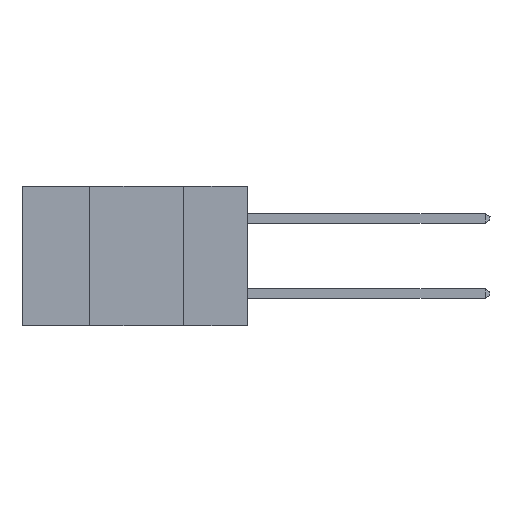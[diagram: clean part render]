
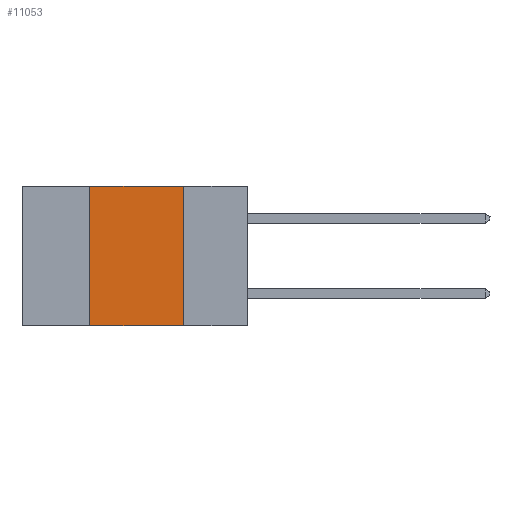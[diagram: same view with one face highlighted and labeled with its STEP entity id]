
A CAD part, left-side view. The second image highlights one B-rep face of the part: STEP entity #11053.
In plain terms, the highlighted planar face has unit normal (-1, 0, 0).
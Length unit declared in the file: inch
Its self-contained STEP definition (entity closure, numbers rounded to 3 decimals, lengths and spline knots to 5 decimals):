
#261 = DIRECTION ( 'NONE',  ( 0., -1., 0. ) ) ;
#822 = CARTESIAN_POINT ( 'NONE',  ( 0., 0.42, 0. ) ) ;
#1198 = VECTOR ( 'NONE', #261, 39.37008 ) ;
#1407 = DIRECTION ( 'NONE',  ( 0., 0., -1. ) ) ;
#1508 = EDGE_CURVE ( 'NONE', #2218, #7993, #6238, .T. ) ;
#2218 = VERTEX_POINT ( 'NONE', #10635 ) ;
#2690 = VECTOR ( 'NONE', #10118, 39.37008 ) ;
#2899 = LINE ( 'NONE', #6430, #2690 ) ;
#2965 = ORIENTED_EDGE ( 'NONE', *, *, #9736, .F. ) ;
#3359 = DIRECTION ( 'NONE',  ( 0., 0., 1. ) ) ;
#4343 = AXIS2_PLACEMENT_3D ( 'NONE', #10699, #7095, #15680 ) ;
#4502 = VERTEX_POINT ( 'NONE', #822 ) ;
#4747 = EDGE_CURVE ( 'NONE', #8510, #7993, #2899, .T. ) ;
#5065 = EDGE_CURVE ( 'NONE', #4502, #2218, #14714, .T. ) ;
#6238 = LINE ( 'NONE', #11136, #9952 ) ;
#6390 = ORIENTED_EDGE ( 'NONE', *, *, #1508, .F. ) ;
#6430 = CARTESIAN_POINT ( 'NONE',  ( 0., 0.6, -0.37 ) ) ;
#6575 = VECTOR ( 'NONE', #3359, 39.37008 ) ;
#6958 = LINE ( 'NONE', #9565, #6575 ) ;
#7030 = ORIENTED_EDGE ( 'NONE', *, *, #4747, .T. ) ;
#7095 = DIRECTION ( 'NONE',  ( 1., 0., 0. ) ) ;
#7584 = CARTESIAN_POINT ( 'NONE',  ( 0., 0.6, 0. ) ) ;
#7993 = VERTEX_POINT ( 'NONE', #9257 ) ;
#8510 = VERTEX_POINT ( 'NONE', #11904 ) ;
#9257 = CARTESIAN_POINT ( 'NONE',  ( 0., 0.17, -0.37 ) ) ;
#9565 = CARTESIAN_POINT ( 'NONE',  ( 0., 0.42, -0.37 ) ) ;
#9736 = EDGE_CURVE ( 'NONE', #8510, #4502, #6958, .T. ) ;
#9952 = VECTOR ( 'NONE', #1407, 39.37008 ) ;
#10118 = DIRECTION ( 'NONE',  ( 0., -1., 0. ) ) ;
#10135 = FACE_OUTER_BOUND ( 'NONE', #10412, .T. ) ;
#10412 = EDGE_LOOP ( 'NONE', ( #6390, #12869, #2965, #7030 ) ) ;
#10635 = CARTESIAN_POINT ( 'NONE',  ( 0., 0.17, 0. ) ) ;
#10699 = CARTESIAN_POINT ( 'NONE',  ( 0., 0.6, 0. ) ) ;
#11053 = ADVANCED_FACE ( 'NONE', ( #10135 ), #11745, .F. ) ;
#11136 = CARTESIAN_POINT ( 'NONE',  ( 0., 0.17, -0.37 ) ) ;
#11745 = PLANE ( 'NONE',  #4343 ) ;
#11904 = CARTESIAN_POINT ( 'NONE',  ( 0., 0.42, -0.37 ) ) ;
#12869 = ORIENTED_EDGE ( 'NONE', *, *, #5065, .F. ) ;
#14714 = LINE ( 'NONE', #7584, #1198 ) ;
#15680 = DIRECTION ( 'NONE',  ( 0., 0., -1. ) ) ;
